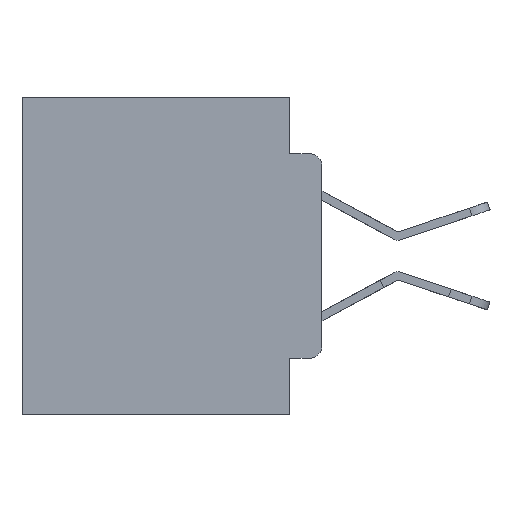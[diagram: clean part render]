
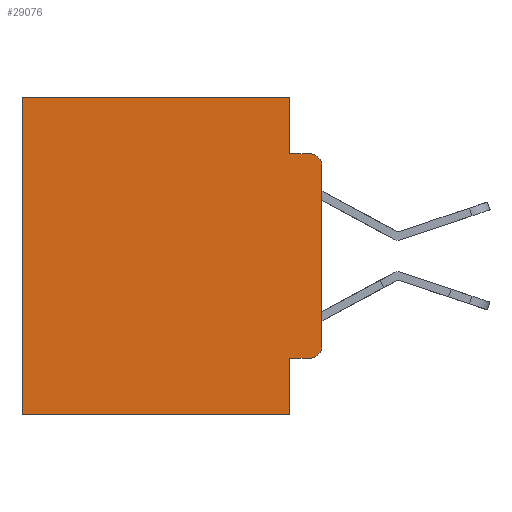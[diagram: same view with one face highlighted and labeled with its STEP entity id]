
A CAD part, left-side view. The second image highlights one B-rep face of the part: STEP entity #29076.
In plain terms, the highlighted planar face has unit normal (-1, 0, 0).
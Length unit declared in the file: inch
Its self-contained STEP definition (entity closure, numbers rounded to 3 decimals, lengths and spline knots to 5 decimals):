
#791 = LINE ( 'NONE', #11249, #19126 ) ;
#1319 = ORIENTED_EDGE ( 'NONE', *, *, #25137, .F. ) ;
#1350 = ORIENTED_EDGE ( 'NONE', *, *, #11057, .T. ) ;
#1363 = CARTESIAN_POINT ( 'NONE',  ( 0.298, 0.051, -0.4115 ) ) ;
#2027 = VECTOR ( 'NONE', #3974, 39.37008 ) ;
#2355 = CARTESIAN_POINT ( 'NONE',  ( 0.298, 0.473, 0. ) ) ;
#2402 = AXIS2_PLACEMENT_3D ( 'NONE', #6326, #22178, #8656 ) ;
#2781 = AXIS2_PLACEMENT_3D ( 'NONE', #24596, #29140, #15780 ) ;
#2804 = VERTEX_POINT ( 'NONE', #15006 ) ;
#2946 = CARTESIAN_POINT ( 'NONE',  ( 0.298, 0., -0.1085 ) ) ;
#3297 = EDGE_CURVE ( 'NONE', #21727, #5387, #12011, .T. ) ;
#3299 = CIRCLE ( 'NONE', #2402, 0.02 ) ;
#3974 = DIRECTION ( 'NONE',  ( 0., 0., -1. ) ) ;
#4188 = VECTOR ( 'NONE', #20605, 39.37008 ) ;
#4558 = DIRECTION ( 'NONE',  ( 0., -1., 0. ) ) ;
#4839 = EDGE_CURVE ( 'NONE', #10009, #21727, #15087, .T. ) ;
#5050 = ORIENTED_EDGE ( 'NONE', *, *, #29261, .T. ) ;
#5387 = VERTEX_POINT ( 'NONE', #12014 ) ;
#5573 = ORIENTED_EDGE ( 'NONE', *, *, #21967, .F. ) ;
#5801 = DIRECTION ( 'NONE',  ( 0., 0., -1. ) ) ;
#5868 = VECTOR ( 'NONE', #13511, 39.37008 ) ;
#5880 = LINE ( 'NONE', #12604, #29143 ) ;
#6326 = CARTESIAN_POINT ( 'NONE',  ( 0.298, 0.02, -0.1085 ) ) ;
#6596 = PLANE ( 'NONE',  #2781 ) ;
#6812 = AXIS2_PLACEMENT_3D ( 'NONE', #8389, #24175, #10741 ) ;
#7175 = CARTESIAN_POINT ( 'NONE',  ( 0.298, 0.051, 0. ) ) ;
#7410 = VERTEX_POINT ( 'NONE', #14024 ) ;
#8152 = ORIENTED_EDGE ( 'NONE', *, *, #4839, .F. ) ;
#8297 = VECTOR ( 'NONE', #24346, 39.37008 ) ;
#8356 = EDGE_LOOP ( 'NONE', ( #10594, #1350, #22157, #8152, #5050, #27033, #5573, #1319, #13313, #22084 ) ) ;
#8389 = CARTESIAN_POINT ( 'NONE',  ( 0.298, 0.02, -0.3915 ) ) ;
#8656 = DIRECTION ( 'NONE',  ( 0., 0., -1. ) ) ;
#10009 = VERTEX_POINT ( 'NONE', #7175 ) ;
#10594 = ORIENTED_EDGE ( 'NONE', *, *, #17070, .F. ) ;
#10741 = DIRECTION ( 'NONE',  ( 0., 0., -1. ) ) ;
#11057 = EDGE_CURVE ( 'NONE', #14808, #5387, #3299, .T. ) ;
#11249 = CARTESIAN_POINT ( 'NONE',  ( 0.298, 0., -0.5 ) ) ;
#12011 = LINE ( 'NONE', #29367, #5868 ) ;
#12014 = CARTESIAN_POINT ( 'NONE',  ( 0.298, 0.02, -0.0885 ) ) ;
#12604 = CARTESIAN_POINT ( 'NONE',  ( 0.298, 0., 0. ) ) ;
#13136 = CARTESIAN_POINT ( 'NONE',  ( 0.298, 0., 0. ) ) ;
#13313 = ORIENTED_EDGE ( 'NONE', *, *, #23645, .T. ) ;
#13511 = DIRECTION ( 'NONE',  ( 0., -1., 0. ) ) ;
#14024 = CARTESIAN_POINT ( 'NONE',  ( 0.298, 0.473, -0.5 ) ) ;
#14808 = VERTEX_POINT ( 'NONE', #2946 ) ;
#15006 = CARTESIAN_POINT ( 'NONE',  ( 0.298, 0.02, -0.4115 ) ) ;
#15087 = LINE ( 'NONE', #20224, #8297 ) ;
#15780 = DIRECTION ( 'NONE',  ( 0., 0., -1. ) ) ;
#15881 = LINE ( 'NONE', #15966, #27089 ) ;
#15966 = CARTESIAN_POINT ( 'NONE',  ( 0.298, 0.051, -0.4115 ) ) ;
#16119 = LINE ( 'NONE', #19398, #22064 ) ;
#17070 = EDGE_CURVE ( 'NONE', #14808, #17894, #20947, .T. ) ;
#17633 = EDGE_CURVE ( 'NONE', #2804, #17894, #24086, .T. ) ;
#17828 = CARTESIAN_POINT ( 'NONE',  ( 0.298, 0.473, 0. ) ) ;
#17894 = VERTEX_POINT ( 'NONE', #23775 ) ;
#19126 = VECTOR ( 'NONE', #26930, 39.37008 ) ;
#19398 = CARTESIAN_POINT ( 'NONE',  ( 0.298, 0.051, 0. ) ) ;
#20224 = CARTESIAN_POINT ( 'NONE',  ( 0.298, 0.051, 0. ) ) ;
#20605 = DIRECTION ( 'NONE',  ( 0., 0., -1. ) ) ;
#20947 = LINE ( 'NONE', #13136, #2027 ) ;
#21727 = VERTEX_POINT ( 'NONE', #23813 ) ;
#21967 = EDGE_CURVE ( 'NONE', #25887, #7410, #791, .T. ) ;
#22064 = VECTOR ( 'NONE', #5801, 39.37008 ) ;
#22084 = ORIENTED_EDGE ( 'NONE', *, *, #17633, .T. ) ;
#22157 = ORIENTED_EDGE ( 'NONE', *, *, #3297, .F. ) ;
#22178 = DIRECTION ( 'NONE',  ( -1., 0., 0. ) ) ;
#23645 = EDGE_CURVE ( 'NONE', #27025, #2804, #15881, .T. ) ;
#23775 = CARTESIAN_POINT ( 'NONE',  ( 0.298, 0., -0.3915 ) ) ;
#23813 = CARTESIAN_POINT ( 'NONE',  ( 0.298, 0.051, -0.0885 ) ) ;
#24086 = CIRCLE ( 'NONE', #6812, 0.02 ) ;
#24175 = DIRECTION ( 'NONE',  ( -1., 0., 0. ) ) ;
#24346 = DIRECTION ( 'NONE',  ( 0., 0., -1. ) ) ;
#24596 = CARTESIAN_POINT ( 'NONE',  ( 0.298, 0., 0. ) ) ;
#25137 = EDGE_CURVE ( 'NONE', #27025, #25887, #16119, .T. ) ;
#25887 = VERTEX_POINT ( 'NONE', #26419 ) ;
#26419 = CARTESIAN_POINT ( 'NONE',  ( 0.298, 0.051, -0.5 ) ) ;
#26652 = EDGE_CURVE ( 'NONE', #27128, #7410, #27550, .T. ) ;
#26930 = DIRECTION ( 'NONE',  ( 0., 1., 0. ) ) ;
#27025 = VERTEX_POINT ( 'NONE', #1363 ) ;
#27033 = ORIENTED_EDGE ( 'NONE', *, *, #26652, .T. ) ;
#27089 = VECTOR ( 'NONE', #4558, 39.37008 ) ;
#27128 = VERTEX_POINT ( 'NONE', #17828 ) ;
#27550 = LINE ( 'NONE', #2355, #4188 ) ;
#28242 = DIRECTION ( 'NONE',  ( 0., 1., 0. ) ) ;
#28814 = FACE_OUTER_BOUND ( 'NONE', #8356, .T. ) ;
#29076 = ADVANCED_FACE ( 'NONE', ( #28814 ), #6596, .F. ) ;
#29140 = DIRECTION ( 'NONE',  ( 1., 0., 0. ) ) ;
#29143 = VECTOR ( 'NONE', #28242, 39.37008 ) ;
#29261 = EDGE_CURVE ( 'NONE', #10009, #27128, #5880, .T. ) ;
#29367 = CARTESIAN_POINT ( 'NONE',  ( 0.298, 0.051, -0.0885 ) ) ;
